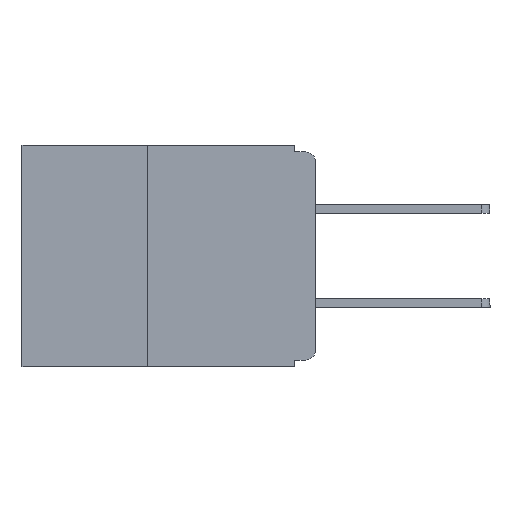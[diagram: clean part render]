
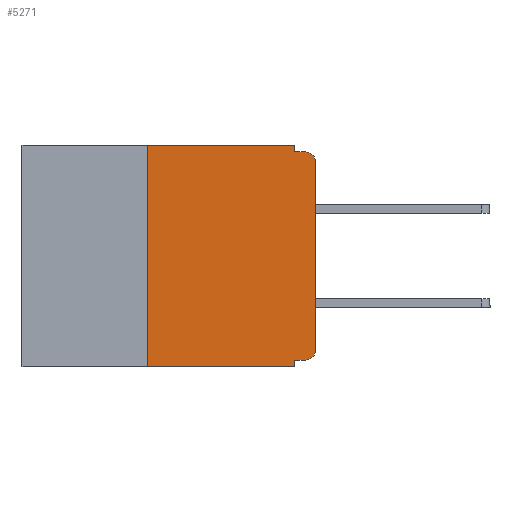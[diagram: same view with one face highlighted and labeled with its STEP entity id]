
A CAD part, left-side view. The second image highlights one B-rep face of the part: STEP entity #5271.
In plain terms, the highlighted planar face has unit normal (-1, 0, 0).
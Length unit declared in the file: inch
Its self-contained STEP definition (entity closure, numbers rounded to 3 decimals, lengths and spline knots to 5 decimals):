
#25 = VECTOR ( 'NONE', #17573, 39.37008 ) ;
#646 = DIRECTION ( 'NONE',  ( -1., 0., 0. ) ) ;
#787 = CARTESIAN_POINT ( 'NONE',  ( 0., 0.437, -0.33 ) ) ;
#835 = LINE ( 'NONE', #20454, #9414 ) ;
#971 = VERTEX_POINT ( 'NONE', #4811 ) ;
#1170 = EDGE_CURVE ( 'NONE', #971, #2009, #4164, .T. ) ;
#1200 = DIRECTION ( 'NONE',  ( 0., -1., 0. ) ) ;
#1311 = FACE_OUTER_BOUND ( 'NONE', #6042, .T. ) ;
#1425 = VERTEX_POINT ( 'NONE', #5947 ) ;
#1515 = DIRECTION ( 'NONE',  ( 0., 0., -1. ) ) ;
#1543 = CARTESIAN_POINT ( 'NONE',  ( 0., 0.25, 0. ) ) ;
#1553 = VECTOR ( 'NONE', #1200, 39.37008 ) ;
#1588 = DIRECTION ( 'NONE',  ( -1., 0., 0. ) ) ;
#1638 = CARTESIAN_POINT ( 'NONE',  ( 0., 0.015, -0.025 ) ) ;
#2009 = VERTEX_POINT ( 'NONE', #1543 ) ;
#2676 = EDGE_CURVE ( 'NONE', #21356, #15259, #835, .T. ) ;
#3492 = CIRCLE ( 'NONE', #6494, 0.015 ) ;
#4085 = CARTESIAN_POINT ( 'NONE',  ( 0., 0., -0.01 ) ) ;
#4106 = VERTEX_POINT ( 'NONE', #11205 ) ;
#4164 = LINE ( 'NONE', #4495, #8723 ) ;
#4236 = VERTEX_POINT ( 'NONE', #9272 ) ;
#4495 = CARTESIAN_POINT ( 'NONE',  ( 0., 0.25, -0.33 ) ) ;
#4619 = DIRECTION ( 'NONE',  ( 0., 0., 1. ) ) ;
#4646 = AXIS2_PLACEMENT_3D ( 'NONE', #14411, #13835, #13567 ) ;
#4811 = CARTESIAN_POINT ( 'NONE',  ( 0., 0.25, -0.33 ) ) ;
#5271 = ADVANCED_FACE ( 'NONE', ( #1311 ), #13904, .F. ) ;
#5543 = ORIENTED_EDGE ( 'NONE', *, *, #5608, .T. ) ;
#5608 = EDGE_CURVE ( 'NONE', #19507, #4236, #3492, .T. ) ;
#5790 = CIRCLE ( 'NONE', #15340, 0.015 ) ;
#5810 = ORIENTED_EDGE ( 'NONE', *, *, #2676, .F. ) ;
#5947 = CARTESIAN_POINT ( 'NONE',  ( 0., 0.031, -0.01 ) ) ;
#6042 = EDGE_LOOP ( 'NONE', ( #8464, #5543, #10588, #11083, #21033, #8756, #17650, #5810, #15823, #11923 ) ) ;
#6494 = AXIS2_PLACEMENT_3D ( 'NONE', #1638, #1588, #1515 ) ;
#6974 = CARTESIAN_POINT ( 'NONE',  ( 0., 0.015, -0.32 ) ) ;
#7693 = VERTEX_POINT ( 'NONE', #16321 ) ;
#8242 = EDGE_CURVE ( 'NONE', #971, #15259, #20751, .T. ) ;
#8349 = CARTESIAN_POINT ( 'NONE',  ( 0., 0., -0.32 ) ) ;
#8464 = ORIENTED_EDGE ( 'NONE', *, *, #10241, .T. ) ;
#8723 = VECTOR ( 'NONE', #4619, 39.37008 ) ;
#8756 = ORIENTED_EDGE ( 'NONE', *, *, #1170, .F. ) ;
#9067 = EDGE_CURVE ( 'NONE', #7693, #1425, #13687, .T. ) ;
#9272 = CARTESIAN_POINT ( 'NONE',  ( 0., 0.015, -0.01 ) ) ;
#9414 = VECTOR ( 'NONE', #20203, 39.37008 ) ;
#10056 = DIRECTION ( 'NONE',  ( 0., 1., 0. ) ) ;
#10241 = EDGE_CURVE ( 'NONE', #4106, #19507, #21188, .T. ) ;
#10588 = ORIENTED_EDGE ( 'NONE', *, *, #13546, .F. ) ;
#10882 = CARTESIAN_POINT ( 'NONE',  ( 0., 0.015, -0.305 ) ) ;
#11083 = ORIENTED_EDGE ( 'NONE', *, *, #9067, .F. ) ;
#11205 = CARTESIAN_POINT ( 'NONE',  ( 0., 0., -0.305 ) ) ;
#11422 = CARTESIAN_POINT ( 'NONE',  ( 0., 0.437, 0. ) ) ;
#11508 = CARTESIAN_POINT ( 'NONE',  ( 0., 0.031, -0.32 ) ) ;
#11923 = ORIENTED_EDGE ( 'NONE', *, *, #19066, .T. ) ;
#11952 = CARTESIAN_POINT ( 'NONE',  ( 0., 0., 0. ) ) ;
#12587 = DIRECTION ( 'NONE',  ( 0., 0., -1. ) ) ;
#13159 = VECTOR ( 'NONE', #18812, 39.37008 ) ;
#13546 = EDGE_CURVE ( 'NONE', #1425, #4236, #14121, .T. ) ;
#13567 = DIRECTION ( 'NONE',  ( 0., 0., -1. ) ) ;
#13687 = LINE ( 'NONE', #13742, #13159 ) ;
#13742 = CARTESIAN_POINT ( 'NONE',  ( 0., 0.031, 0. ) ) ;
#13835 = DIRECTION ( 'NONE',  ( 1., 0., 0. ) ) ;
#13904 = PLANE ( 'NONE',  #4646 ) ;
#14121 = LINE ( 'NONE', #4085, #25 ) ;
#14411 = CARTESIAN_POINT ( 'NONE',  ( 0., 0.437, 0. ) ) ;
#14789 = VECTOR ( 'NONE', #10056, 39.37008 ) ;
#14918 = VERTEX_POINT ( 'NONE', #6974 ) ;
#15226 = DIRECTION ( 'NONE',  ( 0., 0., 1. ) ) ;
#15259 = VERTEX_POINT ( 'NONE', #19707 ) ;
#15340 = AXIS2_PLACEMENT_3D ( 'NONE', #10882, #646, #12587 ) ;
#15823 = ORIENTED_EDGE ( 'NONE', *, *, #18123, .F. ) ;
#15912 = EDGE_CURVE ( 'NONE', #2009, #7693, #19055, .T. ) ;
#16053 = DIRECTION ( 'NONE',  ( 0., -1., 0. ) ) ;
#16237 = VECTOR ( 'NONE', #15226, 39.37008 ) ;
#16321 = CARTESIAN_POINT ( 'NONE',  ( 0., 0.031, 0. ) ) ;
#17573 = DIRECTION ( 'NONE',  ( 0., -1., 0. ) ) ;
#17650 = ORIENTED_EDGE ( 'NONE', *, *, #8242, .T. ) ;
#18123 = EDGE_CURVE ( 'NONE', #14918, #21356, #18749, .T. ) ;
#18734 = CARTESIAN_POINT ( 'NONE',  ( 0., 0., -0.025 ) ) ;
#18749 = LINE ( 'NONE', #8349, #14789 ) ;
#18812 = DIRECTION ( 'NONE',  ( 0., 0., -1. ) ) ;
#19055 = LINE ( 'NONE', #11422, #1553 ) ;
#19066 = EDGE_CURVE ( 'NONE', #14918, #4106, #5790, .T. ) ;
#19507 = VERTEX_POINT ( 'NONE', #18734 ) ;
#19707 = CARTESIAN_POINT ( 'NONE',  ( 0., 0.031, -0.33 ) ) ;
#20203 = DIRECTION ( 'NONE',  ( 0., 0., -1. ) ) ;
#20218 = VECTOR ( 'NONE', #16053, 39.37008 ) ;
#20454 = CARTESIAN_POINT ( 'NONE',  ( 0., 0.031, -0.33 ) ) ;
#20751 = LINE ( 'NONE', #787, #20218 ) ;
#21033 = ORIENTED_EDGE ( 'NONE', *, *, #15912, .F. ) ;
#21188 = LINE ( 'NONE', #11952, #16237 ) ;
#21356 = VERTEX_POINT ( 'NONE', #11508 ) ;
